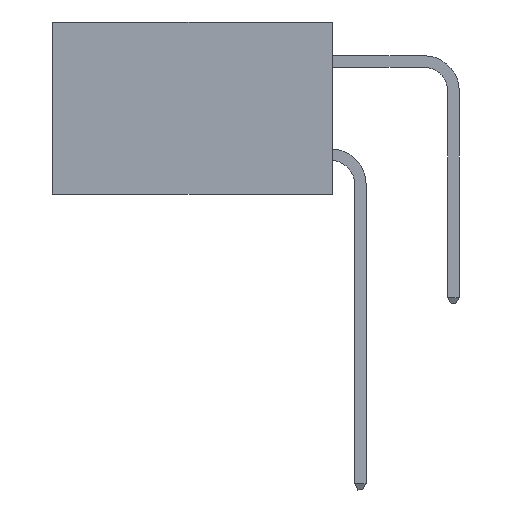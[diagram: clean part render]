
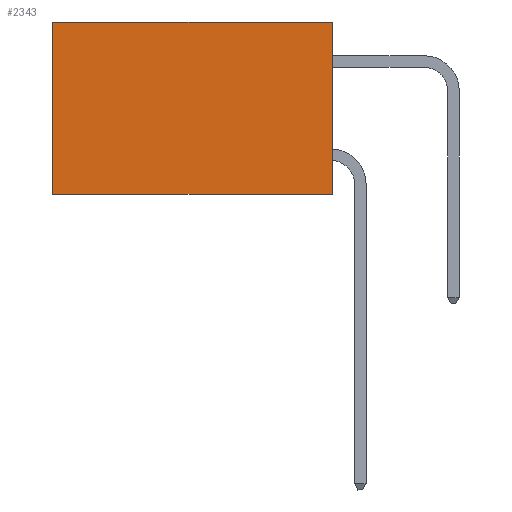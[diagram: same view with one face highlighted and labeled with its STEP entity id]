
A CAD part, left-side view. The second image highlights one B-rep face of the part: STEP entity #2343.
In plain terms, the highlighted planar face has unit normal (-1, 0, 0).
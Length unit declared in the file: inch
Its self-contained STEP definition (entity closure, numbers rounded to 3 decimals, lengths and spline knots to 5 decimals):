
#182 = EDGE_CURVE ( 'NONE', #14502, #19164, #7015, .T. ) ;
#757 = CARTESIAN_POINT ( 'NONE',  ( 0.2615, 0.6, -0.37 ) ) ;
#1189 = ORIENTED_EDGE ( 'NONE', *, *, #182, .T. ) ;
#1897 = FACE_OUTER_BOUND ( 'NONE', #18330, .T. ) ;
#2343 = ADVANCED_FACE ( 'NONE', ( #1897 ), #9987, .F. ) ;
#2589 = CARTESIAN_POINT ( 'NONE',  ( 0.2615, 0.6, 0. ) ) ;
#2822 = EDGE_CURVE ( 'NONE', #3233, #2959, #11370, .T. ) ;
#2959 = VERTEX_POINT ( 'NONE', #10671 ) ;
#3233 = VERTEX_POINT ( 'NONE', #11593 ) ;
#3395 = CARTESIAN_POINT ( 'NONE',  ( 0.2615, 0., -0.37 ) ) ;
#4704 = LINE ( 'NONE', #11611, #19789 ) ;
#5383 = DIRECTION ( 'NONE',  ( 0., 0., -1. ) ) ;
#6421 = VECTOR ( 'NONE', #18065, 39.37008 ) ;
#7015 = LINE ( 'NONE', #12507, #6421 ) ;
#7328 = ORIENTED_EDGE ( 'NONE', *, *, #19204, .T. ) ;
#7450 = VECTOR ( 'NONE', #19724, 39.37008 ) ;
#9461 = EDGE_CURVE ( 'NONE', #2959, #19164, #4704, .T. ) ;
#9987 = PLANE ( 'NONE',  #14428 ) ;
#10291 = CARTESIAN_POINT ( 'NONE',  ( 0.2615, 0., 0. ) ) ;
#10619 = ORIENTED_EDGE ( 'NONE', *, *, #9461, .F. ) ;
#10671 = CARTESIAN_POINT ( 'NONE',  ( 0.2615, 0., -0.37 ) ) ;
#11370 = LINE ( 'NONE', #3395, #21982 ) ;
#11593 = CARTESIAN_POINT ( 'NONE',  ( 0.2615, 0., 0. ) ) ;
#11611 = CARTESIAN_POINT ( 'NONE',  ( 0.2615, 0., -0.37 ) ) ;
#11701 = DIRECTION ( 'NONE',  ( 0., 1., 0. ) ) ;
#12507 = CARTESIAN_POINT ( 'NONE',  ( 0.2615, 0.6, -0.37 ) ) ;
#12571 = DIRECTION ( 'NONE',  ( 0., 0., -1. ) ) ;
#14428 = AXIS2_PLACEMENT_3D ( 'NONE', #21444, #21365, #5383 ) ;
#14502 = VERTEX_POINT ( 'NONE', #2589 ) ;
#17493 = LINE ( 'NONE', #10291, #7450 ) ;
#17760 = ORIENTED_EDGE ( 'NONE', *, *, #2822, .F. ) ;
#18065 = DIRECTION ( 'NONE',  ( 0., 0., -1. ) ) ;
#18330 = EDGE_LOOP ( 'NONE', ( #1189, #10619, #17760, #7328 ) ) ;
#19164 = VERTEX_POINT ( 'NONE', #757 ) ;
#19204 = EDGE_CURVE ( 'NONE', #3233, #14502, #17493, .T. ) ;
#19724 = DIRECTION ( 'NONE',  ( 0., 1., 0. ) ) ;
#19789 = VECTOR ( 'NONE', #11701, 39.37008 ) ;
#21365 = DIRECTION ( 'NONE',  ( 1., 0., 0. ) ) ;
#21444 = CARTESIAN_POINT ( 'NONE',  ( 0.2615, 0., -0.37 ) ) ;
#21982 = VECTOR ( 'NONE', #12571, 39.37008 ) ;
